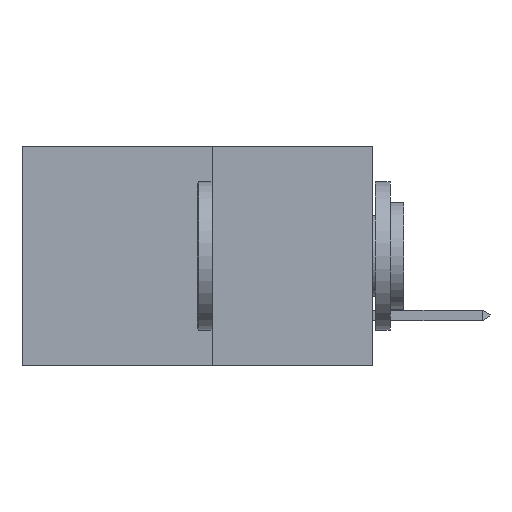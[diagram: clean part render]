
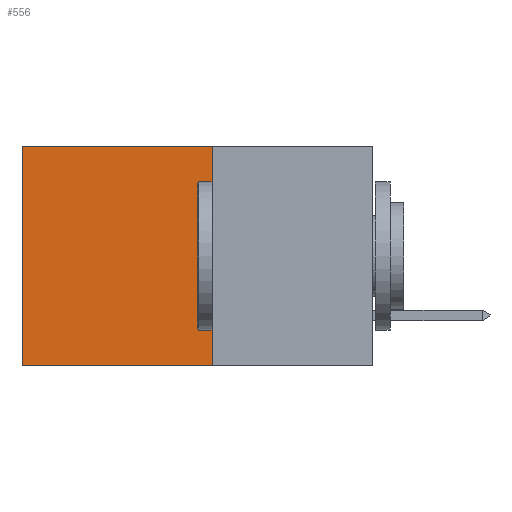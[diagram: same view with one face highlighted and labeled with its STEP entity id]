
A CAD part, left-side view. The second image highlights one B-rep face of the part: STEP entity #556.
In plain terms, the highlighted planar face has unit normal (-1, 0, 0).
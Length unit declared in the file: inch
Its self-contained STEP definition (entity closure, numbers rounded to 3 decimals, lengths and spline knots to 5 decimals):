
#556 = ADVANCED_FACE ( 'NONE', ( #12347 ), #23291, .F. ) ;
#814 = VERTEX_POINT ( 'NONE', #21242 ) ;
#2959 = VECTOR ( 'NONE', #28070, 39.37008 ) ;
#3591 = DIRECTION ( 'NONE',  ( 0., 1., 0. ) ) ;
#3625 = CARTESIAN_POINT ( 'NONE',  ( 0.277, 0.27, -0.37 ) ) ;
#3727 = CARTESIAN_POINT ( 'NONE',  ( 0.277, 0.27, -0.37 ) ) ;
#4530 = EDGE_CURVE ( 'NONE', #6010, #15869, #14951, .T. ) ;
#6010 = VERTEX_POINT ( 'NONE', #18320 ) ;
#7879 = DIRECTION ( 'NONE',  ( 0., 0., -1. ) ) ;
#9948 = LINE ( 'NONE', #16739, #23192 ) ;
#9974 = EDGE_LOOP ( 'NONE', ( #23596, #17150, #25593, #21217 ) ) ;
#9981 = LINE ( 'NONE', #14848, #2959 ) ;
#12347 = FACE_OUTER_BOUND ( 'NONE', #9974, .T. ) ;
#14120 = VECTOR ( 'NONE', #16075, 39.37008 ) ;
#14221 = EDGE_CURVE ( 'NONE', #6010, #20452, #21370, .T. ) ;
#14352 = VECTOR ( 'NONE', #24769, 39.37008 ) ;
#14848 = CARTESIAN_POINT ( 'NONE',  ( 0.277, 0.59, -0.37 ) ) ;
#14863 = DIRECTION ( 'NONE',  ( 1., 0., 0. ) ) ;
#14951 = LINE ( 'NONE', #16521, #14120 ) ;
#15869 = VERTEX_POINT ( 'NONE', #26845 ) ;
#16075 = DIRECTION ( 'NONE',  ( 0., 1., 0. ) ) ;
#16521 = CARTESIAN_POINT ( 'NONE',  ( 0.277, 0.27, 0. ) ) ;
#16739 = CARTESIAN_POINT ( 'NONE',  ( 0.277, 0.27, -0.37 ) ) ;
#17150 = ORIENTED_EDGE ( 'NONE', *, *, #28281, .F. ) ;
#18320 = CARTESIAN_POINT ( 'NONE',  ( 0.277, 0.27, 0. ) ) ;
#20452 = VERTEX_POINT ( 'NONE', #29589 ) ;
#21217 = ORIENTED_EDGE ( 'NONE', *, *, #4530, .T. ) ;
#21242 = CARTESIAN_POINT ( 'NONE',  ( 0.277, 0.59, -0.37 ) ) ;
#21370 = LINE ( 'NONE', #3625, #14352 ) ;
#22139 = AXIS2_PLACEMENT_3D ( 'NONE', #3727, #14863, #7879 ) ;
#23192 = VECTOR ( 'NONE', #3591, 39.37008 ) ;
#23291 = PLANE ( 'NONE',  #22139 ) ;
#23596 = ORIENTED_EDGE ( 'NONE', *, *, #27834, .T. ) ;
#24769 = DIRECTION ( 'NONE',  ( 0., 0., -1. ) ) ;
#25593 = ORIENTED_EDGE ( 'NONE', *, *, #14221, .F. ) ;
#26845 = CARTESIAN_POINT ( 'NONE',  ( 0.277, 0.59, 0. ) ) ;
#27834 = EDGE_CURVE ( 'NONE', #15869, #814, #9981, .T. ) ;
#28070 = DIRECTION ( 'NONE',  ( 0., 0., -1. ) ) ;
#28281 = EDGE_CURVE ( 'NONE', #20452, #814, #9948, .T. ) ;
#29589 = CARTESIAN_POINT ( 'NONE',  ( 0.277, 0.27, -0.37 ) ) ;
